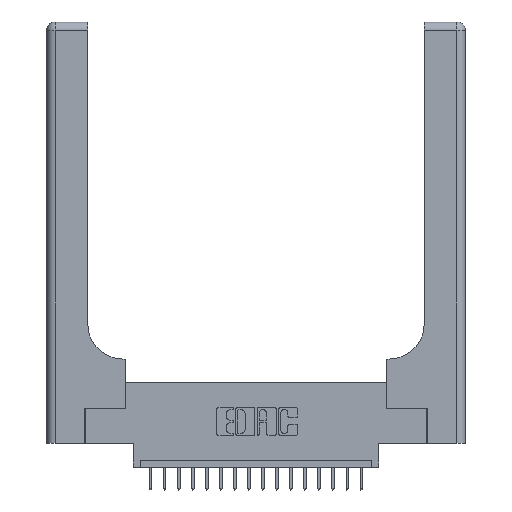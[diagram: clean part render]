
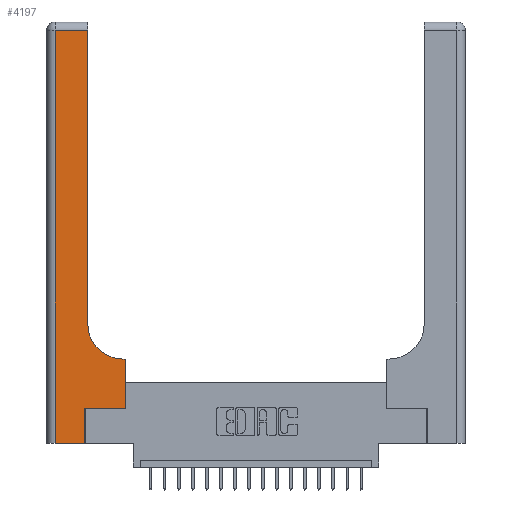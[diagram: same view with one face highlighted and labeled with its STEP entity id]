
A CAD part, top view. The second image highlights one B-rep face of the part: STEP entity #4197.
In plain terms, the highlighted planar face has unit normal (0, 0, 1).
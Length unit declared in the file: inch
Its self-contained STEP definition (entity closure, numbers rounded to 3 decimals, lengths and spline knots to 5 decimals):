
#223 = CARTESIAN_POINT ( 'NONE',  ( 0.06, 3., 0.37 ) ) ;
#354 = CARTESIAN_POINT ( 'NONE',  ( 0., 3., 0.37 ) ) ;
#1725 = DIRECTION ( 'NONE',  ( 1., 0., 0. ) ) ;
#1766 = CARTESIAN_POINT ( 'NONE',  ( 0., 2.94, 0.37 ) ) ;
#1931 = DIRECTION ( 'NONE',  ( -1., 0., 0. ) ) ;
#2748 = DIRECTION ( 'NONE',  ( 1., 0., 0. ) ) ;
#2749 = EDGE_CURVE ( 'NONE', #4353, #17940, #9036, .T. ) ;
#2852 = VECTOR ( 'NONE', #19198, 39.37008 ) ;
#2983 = CARTESIAN_POINT ( 'NONE',  ( 0.06, 0., 0.37 ) ) ;
#3038 = CARTESIAN_POINT ( 'NONE',  ( 0.06, 2.94, 0.37 ) ) ;
#3180 = CARTESIAN_POINT ( 'NONE',  ( 0.5585, 0.25, 0.37 ) ) ;
#3583 = DIRECTION ( 'NONE',  ( 0., 0., -1. ) ) ;
#3731 = ORIENTED_EDGE ( 'NONE', *, *, #3994, .T. ) ;
#3965 = CARTESIAN_POINT ( 'NONE',  ( 0.5415, 0.6, 0.37 ) ) ;
#3994 = EDGE_CURVE ( 'NONE', #16665, #7962, #17089, .T. ) ;
#4197 = ADVANCED_FACE ( 'NONE', ( #20116 ), #13174, .F. ) ;
#4353 = VERTEX_POINT ( 'NONE', #3965 ) ;
#4996 = ORIENTED_EDGE ( 'NONE', *, *, #5079, .T. ) ;
#5046 = EDGE_CURVE ( 'NONE', #17940, #18033, #19597, .T. ) ;
#5079 = EDGE_CURVE ( 'NONE', #10015, #16287, #7952, .T. ) ;
#5223 = DIRECTION ( 'NONE',  ( -1., 0., 0. ) ) ;
#5250 = VECTOR ( 'NONE', #1725, 39.37008 ) ;
#6265 = EDGE_CURVE ( 'NONE', #12122, #14810, #10195, .T. ) ;
#6500 = ORIENTED_EDGE ( 'NONE', *, *, #16331, .T. ) ;
#6609 = DIRECTION ( 'NONE',  ( 0., 1., 0. ) ) ;
#6924 = CARTESIAN_POINT ( 'NONE',  ( 0., 0., 0.37 ) ) ;
#7036 = AXIS2_PLACEMENT_3D ( 'NONE', #12567, #11015, #2748 ) ;
#7400 = DIRECTION ( 'NONE',  ( 0., -1., 0. ) ) ;
#7952 = LINE ( 'NONE', #223, #18851 ) ;
#7962 = VERTEX_POINT ( 'NONE', #10873 ) ;
#9036 = CIRCLE ( 'NONE', #7036, 0.25 ) ;
#9115 = ORIENTED_EDGE ( 'NONE', *, *, #19086, .T. ) ;
#9430 = DIRECTION ( 'NONE',  ( 0., 1., 0. ) ) ;
#9549 = LINE ( 'NONE', #19338, #5250 ) ;
#9842 = CARTESIAN_POINT ( 'NONE',  ( 0.2915, 0.6, 0.37 ) ) ;
#10015 = VERTEX_POINT ( 'NONE', #3038 ) ;
#10195 = LINE ( 'NONE', #14374, #2852 ) ;
#10472 = CARTESIAN_POINT ( 'NONE',  ( 0.5585, 0.25, 0.37 ) ) ;
#10873 = CARTESIAN_POINT ( 'NONE',  ( 0.5585, 0.6, 0.37 ) ) ;
#10877 = LINE ( 'NONE', #9842, #20018 ) ;
#11015 = DIRECTION ( 'NONE',  ( 0., 0., -1. ) ) ;
#11037 = VECTOR ( 'NONE', #20830, 39.37008 ) ;
#11443 = ORIENTED_EDGE ( 'NONE', *, *, #2749, .T. ) ;
#12122 = VERTEX_POINT ( 'NONE', #14671 ) ;
#12567 = CARTESIAN_POINT ( 'NONE',  ( 0.5415, 0.85, 0.37 ) ) ;
#12995 = EDGE_CURVE ( 'NONE', #18033, #10015, #14067, .T. ) ;
#13174 = PLANE ( 'NONE',  #13836 ) ;
#13279 = CARTESIAN_POINT ( 'NONE',  ( 0.269, 0.25, 0.37 ) ) ;
#13460 = LINE ( 'NONE', #6924, #19824 ) ;
#13836 = AXIS2_PLACEMENT_3D ( 'NONE', #354, #3583, #5223 ) ;
#14067 = LINE ( 'NONE', #1766, #11037 ) ;
#14099 = ORIENTED_EDGE ( 'NONE', *, *, #5046, .T. ) ;
#14374 = CARTESIAN_POINT ( 'NONE',  ( 0.269, 0., 0.37 ) ) ;
#14622 = CARTESIAN_POINT ( 'NONE',  ( 0.2915, 2.94, 0.37 ) ) ;
#14671 = CARTESIAN_POINT ( 'NONE',  ( 0.269, 0., 0.37 ) ) ;
#14810 = VERTEX_POINT ( 'NONE', #13279 ) ;
#15021 = VECTOR ( 'NONE', #9430, 39.37008 ) ;
#15151 = EDGE_CURVE ( 'NONE', #16287, #12122, #13460, .T. ) ;
#15371 = CARTESIAN_POINT ( 'NONE',  ( 0.2915, 3., 0.37 ) ) ;
#16287 = VERTEX_POINT ( 'NONE', #2983 ) ;
#16331 = EDGE_CURVE ( 'NONE', #7962, #4353, #10877, .T. ) ;
#16665 = VERTEX_POINT ( 'NONE', #3180 ) ;
#17089 = LINE ( 'NONE', #10472, #19134 ) ;
#17465 = EDGE_LOOP ( 'NONE', ( #14099, #20441, #4996, #17864, #17617, #9115, #3731, #6500, #11443 ) ) ;
#17617 = ORIENTED_EDGE ( 'NONE', *, *, #6265, .T. ) ;
#17864 = ORIENTED_EDGE ( 'NONE', *, *, #15151, .T. ) ;
#17892 = CARTESIAN_POINT ( 'NONE',  ( 0.2915, 0.85, 0.37 ) ) ;
#17940 = VERTEX_POINT ( 'NONE', #17892 ) ;
#18033 = VERTEX_POINT ( 'NONE', #14622 ) ;
#18261 = DIRECTION ( 'NONE',  ( 1., 0., 0. ) ) ;
#18851 = VECTOR ( 'NONE', #7400, 39.37008 ) ;
#19086 = EDGE_CURVE ( 'NONE', #14810, #16665, #9549, .T. ) ;
#19134 = VECTOR ( 'NONE', #6609, 39.37008 ) ;
#19198 = DIRECTION ( 'NONE',  ( 0., 1., 0. ) ) ;
#19338 = CARTESIAN_POINT ( 'NONE',  ( 0.269, 0.25, 0.37 ) ) ;
#19597 = LINE ( 'NONE', #15371, #15021 ) ;
#19824 = VECTOR ( 'NONE', #18261, 39.37008 ) ;
#20018 = VECTOR ( 'NONE', #1931, 39.37008 ) ;
#20116 = FACE_OUTER_BOUND ( 'NONE', #17465, .T. ) ;
#20441 = ORIENTED_EDGE ( 'NONE', *, *, #12995, .T. ) ;
#20830 = DIRECTION ( 'NONE',  ( -1., 0., 0. ) ) ;
